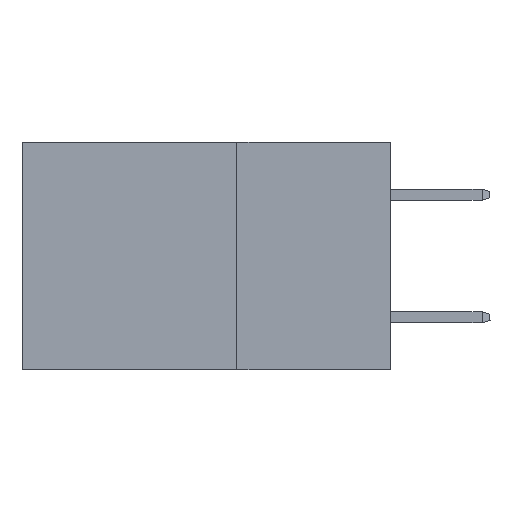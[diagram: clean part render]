
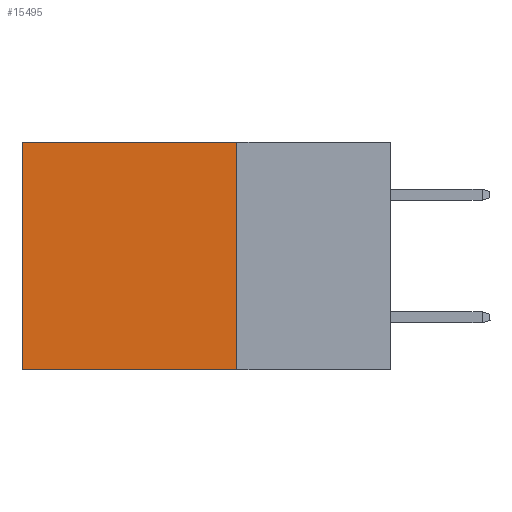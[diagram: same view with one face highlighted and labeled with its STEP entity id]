
A CAD part, left-side view. The second image highlights one B-rep face of the part: STEP entity #15495.
In plain terms, the highlighted planar face has unit normal (-1, 0, 0).
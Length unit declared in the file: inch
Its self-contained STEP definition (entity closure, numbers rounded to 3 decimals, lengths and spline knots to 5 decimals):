
#1231 = EDGE_CURVE ( 'NONE', #41662, #5795, #10762, .T. ) ;
#3603 = CARTESIAN_POINT ( 'NONE',  ( 0.2875, 0.6, -0.37 ) ) ;
#3789 = VECTOR ( 'NONE', #20645, 39.37008 ) ;
#3848 = CARTESIAN_POINT ( 'NONE',  ( 0.2875, 0.25, 0. ) ) ;
#5795 = VERTEX_POINT ( 'NONE', #40087 ) ;
#9001 = CARTESIAN_POINT ( 'NONE',  ( 0.2875, 0.25, -0.37 ) ) ;
#10762 = LINE ( 'NONE', #36879, #36085 ) ;
#11492 = EDGE_CURVE ( 'NONE', #41662, #42024, #31781, .T. ) ;
#11984 = EDGE_CURVE ( 'NONE', #42024, #29773, #38257, .T. ) ;
#12472 = PLANE ( 'NONE',  #22531 ) ;
#12802 = DIRECTION ( 'NONE',  ( 0., 1., 0. ) ) ;
#13142 = ORIENTED_EDGE ( 'NONE', *, *, #31181, .T. ) ;
#15495 = ADVANCED_FACE ( 'NONE', ( #22849 ), #12472, .F. ) ;
#19421 = DIRECTION ( 'NONE',  ( 0., 0., -1. ) ) ;
#20101 = VECTOR ( 'NONE', #21749, 39.37008 ) ;
#20645 = DIRECTION ( 'NONE',  ( 0., 0., -1. ) ) ;
#21158 = LINE ( 'NONE', #25218, #20101 ) ;
#21749 = DIRECTION ( 'NONE',  ( 0., 0., -1. ) ) ;
#22531 = AXIS2_PLACEMENT_3D ( 'NONE', #36562, #40017, #19421 ) ;
#22849 = FACE_OUTER_BOUND ( 'NONE', #29883, .T. ) ;
#25218 = CARTESIAN_POINT ( 'NONE',  ( 0.2875, 0.6, 0. ) ) ;
#27585 = CARTESIAN_POINT ( 'NONE',  ( 0.2875, 0.25, 0. ) ) ;
#29773 = VERTEX_POINT ( 'NONE', #3603 ) ;
#29883 = EDGE_LOOP ( 'NONE', ( #13142, #40253, #38439, #30777 ) ) ;
#30264 = CARTESIAN_POINT ( 'NONE',  ( 0.2875, 0.25, -0.37 ) ) ;
#30777 = ORIENTED_EDGE ( 'NONE', *, *, #1231, .T. ) ;
#31181 = EDGE_CURVE ( 'NONE', #5795, #29773, #21158, .T. ) ;
#31781 = LINE ( 'NONE', #27585, #3789 ) ;
#33705 = DIRECTION ( 'NONE',  ( 0., 1., 0. ) ) ;
#36085 = VECTOR ( 'NONE', #12802, 39.37008 ) ;
#36562 = CARTESIAN_POINT ( 'NONE',  ( 0.2875, 0.25, 0. ) ) ;
#36879 = CARTESIAN_POINT ( 'NONE',  ( 0.2875, 0.25, 0. ) ) ;
#37174 = VECTOR ( 'NONE', #33705, 39.37008 ) ;
#38257 = LINE ( 'NONE', #30264, #37174 ) ;
#38439 = ORIENTED_EDGE ( 'NONE', *, *, #11492, .F. ) ;
#40017 = DIRECTION ( 'NONE',  ( 1., 0., 0. ) ) ;
#40087 = CARTESIAN_POINT ( 'NONE',  ( 0.2875, 0.6, 0. ) ) ;
#40253 = ORIENTED_EDGE ( 'NONE', *, *, #11984, .F. ) ;
#41662 = VERTEX_POINT ( 'NONE', #3848 ) ;
#42024 = VERTEX_POINT ( 'NONE', #9001 ) ;
